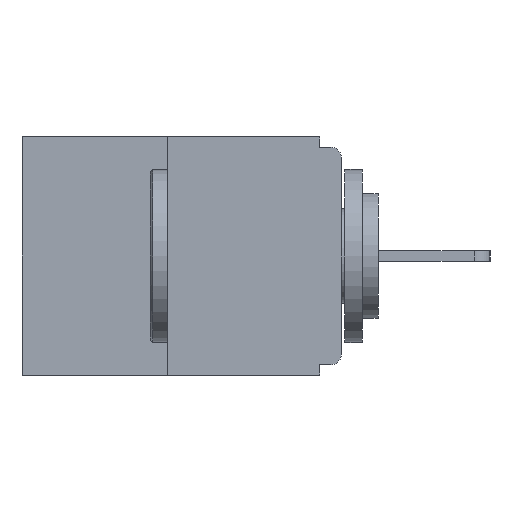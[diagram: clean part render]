
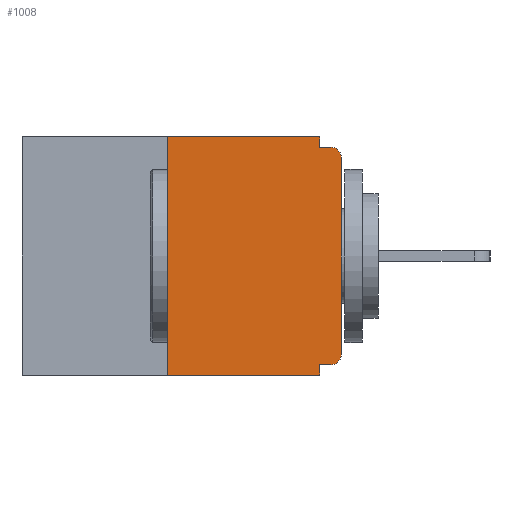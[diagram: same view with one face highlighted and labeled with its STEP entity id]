
A CAD part, left-side view. The second image highlights one B-rep face of the part: STEP entity #1008.
In plain terms, the highlighted planar face has unit normal (-1, 0, 0).
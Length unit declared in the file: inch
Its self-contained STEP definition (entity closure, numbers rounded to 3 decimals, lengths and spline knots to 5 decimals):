
#99 = VECTOR ( 'NONE', #4294, 39.37008 ) ;
#182 = EDGE_CURVE ( 'NONE', #7097, #13514, #10231, .T. ) ;
#261 = CARTESIAN_POINT ( 'NONE',  ( 0., 0., -0.015 ) ) ;
#480 = DIRECTION ( 'NONE',  ( 0., -1., 0. ) ) ;
#609 = DIRECTION ( 'NONE',  ( 0., 0., -1. ) ) ;
#637 = CARTESIAN_POINT ( 'NONE',  ( 0., 0., 0. ) ) ;
#1008 = ADVANCED_FACE ( 'NONE', ( #6346 ), #3076, .F. ) ;
#1031 = ORIENTED_EDGE ( 'NONE', *, *, #1734, .T. ) ;
#1357 = VECTOR ( 'NONE', #10613, 39.37008 ) ;
#1427 = DIRECTION ( 'NONE',  ( 0., 0., -1. ) ) ;
#1679 = CARTESIAN_POINT ( 'NONE',  ( 0., 0.031, -0.015 ) ) ;
#1734 = EDGE_CURVE ( 'NONE', #17250, #7097, #10751, .T. ) ;
#2506 = VECTOR ( 'NONE', #480, 39.37008 ) ;
#3076 = PLANE ( 'NONE',  #16220 ) ;
#3237 = CARTESIAN_POINT ( 'NONE',  ( 0., 0.015, -0.015 ) ) ;
#3392 = EDGE_CURVE ( 'NONE', #21552, #13534, #15521, .T. ) ;
#4152 = ORIENTED_EDGE ( 'NONE', *, *, #4655, .T. ) ;
#4294 = DIRECTION ( 'NONE',  ( 0., -1., 0. ) ) ;
#4646 = VECTOR ( 'NONE', #10646, 39.37008 ) ;
#4655 = EDGE_CURVE ( 'NONE', #6322, #17250, #12391, .T. ) ;
#5084 = ORIENTED_EDGE ( 'NONE', *, *, #21328, .F. ) ;
#5425 = LINE ( 'NONE', #8947, #1357 ) ;
#5510 = EDGE_CURVE ( 'NONE', #9294, #17780, #12289, .T. ) ;
#5581 = LINE ( 'NONE', #10659, #99 ) ;
#5829 = DIRECTION ( 'NONE',  ( -1., 0., 0. ) ) ;
#5840 = CARTESIAN_POINT ( 'NONE',  ( 0., 0.46, 0. ) ) ;
#5875 = ORIENTED_EDGE ( 'NONE', *, *, #19578, .F. ) ;
#6071 = VECTOR ( 'NONE', #9087, 39.37008 ) ;
#6128 = CARTESIAN_POINT ( 'NONE',  ( 0., 0.25, -0.343 ) ) ;
#6322 = VERTEX_POINT ( 'NONE', #21471 ) ;
#6346 = FACE_OUTER_BOUND ( 'NONE', #16700, .T. ) ;
#6513 = CARTESIAN_POINT ( 'NONE',  ( 0., 0.031, 0. ) ) ;
#7097 = VERTEX_POINT ( 'NONE', #9362 ) ;
#7353 = CARTESIAN_POINT ( 'NONE',  ( 0., 0.015, -0.03 ) ) ;
#7396 = AXIS2_PLACEMENT_3D ( 'NONE', #7353, #5829, #18907 ) ;
#7602 = CARTESIAN_POINT ( 'NONE',  ( 0., 0.25, 0. ) ) ;
#7717 = ORIENTED_EDGE ( 'NONE', *, *, #10076, .F. ) ;
#8520 = DIRECTION ( 'NONE',  ( 0., 0., 1. ) ) ;
#8718 = CARTESIAN_POINT ( 'NONE',  ( 0., 0., -0.313 ) ) ;
#8947 = CARTESIAN_POINT ( 'NONE',  ( 0., 0.031, 0. ) ) ;
#9087 = DIRECTION ( 'NONE',  ( 0., 0., -1. ) ) ;
#9138 = ORIENTED_EDGE ( 'NONE', *, *, #14663, .F. ) ;
#9144 = CARTESIAN_POINT ( 'NONE',  ( 0., 0., -0.328 ) ) ;
#9294 = VERTEX_POINT ( 'NONE', #21385 ) ;
#9301 = VECTOR ( 'NONE', #15317, 39.37008 ) ;
#9362 = CARTESIAN_POINT ( 'NONE',  ( 0., 0., -0.03 ) ) ;
#9433 = VECTOR ( 'NONE', #19144, 39.37008 ) ;
#9762 = CARTESIAN_POINT ( 'NONE',  ( 0., 0.46, 0. ) ) ;
#10050 = VECTOR ( 'NONE', #8520, 39.37008 ) ;
#10076 = EDGE_CURVE ( 'NONE', #6322, #9294, #10805, .T. ) ;
#10145 = ORIENTED_EDGE ( 'NONE', *, *, #3392, .F. ) ;
#10231 = CIRCLE ( 'NONE', #7396, 0.015 ) ;
#10294 = AXIS2_PLACEMENT_3D ( 'NONE', #15001, #20047, #609 ) ;
#10613 = DIRECTION ( 'NONE',  ( 0., 0., -1. ) ) ;
#10646 = DIRECTION ( 'NONE',  ( 0., 0., 1. ) ) ;
#10659 = CARTESIAN_POINT ( 'NONE',  ( 0., 0.46, -0.343 ) ) ;
#10751 = LINE ( 'NONE', #637, #4646 ) ;
#10805 = LINE ( 'NONE', #9144, #9433 ) ;
#12289 = LINE ( 'NONE', #17331, #6071 ) ;
#12391 = CIRCLE ( 'NONE', #10294, 0.015 ) ;
#12825 = EDGE_CURVE ( 'NONE', #20684, #17780, #5581, .T. ) ;
#13514 = VERTEX_POINT ( 'NONE', #3237 ) ;
#13534 = VERTEX_POINT ( 'NONE', #6513 ) ;
#14293 = CARTESIAN_POINT ( 'NONE',  ( 0., 0.031, -0.343 ) ) ;
#14663 = EDGE_CURVE ( 'NONE', #18647, #13514, #17068, .T. ) ;
#14874 = ORIENTED_EDGE ( 'NONE', *, *, #182, .T. ) ;
#15001 = CARTESIAN_POINT ( 'NONE',  ( 0., 0.015, -0.313 ) ) ;
#15311 = ORIENTED_EDGE ( 'NONE', *, *, #5510, .F. ) ;
#15317 = DIRECTION ( 'NONE',  ( 0., -1., 0. ) ) ;
#15521 = LINE ( 'NONE', #5840, #2506 ) ;
#16058 = ORIENTED_EDGE ( 'NONE', *, *, #12825, .T. ) ;
#16220 = AXIS2_PLACEMENT_3D ( 'NONE', #9762, #16447, #1427 ) ;
#16447 = DIRECTION ( 'NONE',  ( 1., 0., 0. ) ) ;
#16700 = EDGE_LOOP ( 'NONE', ( #10145, #5875, #16058, #15311, #7717, #4152, #1031, #14874, #9138, #5084 ) ) ;
#17068 = LINE ( 'NONE', #261, #9301 ) ;
#17250 = VERTEX_POINT ( 'NONE', #8718 ) ;
#17331 = CARTESIAN_POINT ( 'NONE',  ( 0., 0.031, -0.343 ) ) ;
#17780 = VERTEX_POINT ( 'NONE', #14293 ) ;
#18633 = LINE ( 'NONE', #20062, #10050 ) ;
#18647 = VERTEX_POINT ( 'NONE', #1679 ) ;
#18907 = DIRECTION ( 'NONE',  ( 0., 0., -1. ) ) ;
#19144 = DIRECTION ( 'NONE',  ( 0., 1., 0. ) ) ;
#19578 = EDGE_CURVE ( 'NONE', #20684, #21552, #18633, .T. ) ;
#20047 = DIRECTION ( 'NONE',  ( -1., 0., 0. ) ) ;
#20062 = CARTESIAN_POINT ( 'NONE',  ( 0., 0.25, 0. ) ) ;
#20684 = VERTEX_POINT ( 'NONE', #6128 ) ;
#21328 = EDGE_CURVE ( 'NONE', #13534, #18647, #5425, .T. ) ;
#21385 = CARTESIAN_POINT ( 'NONE',  ( 0., 0.031, -0.328 ) ) ;
#21471 = CARTESIAN_POINT ( 'NONE',  ( 0., 0.015, -0.328 ) ) ;
#21552 = VERTEX_POINT ( 'NONE', #7602 ) ;
